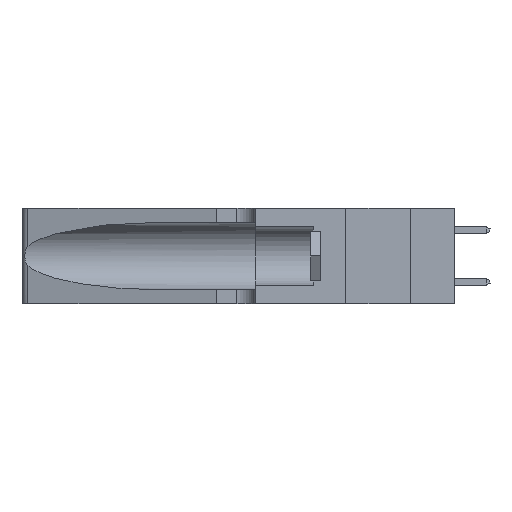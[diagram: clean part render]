
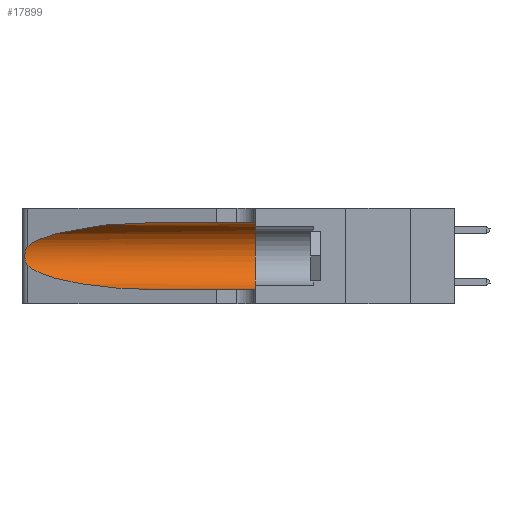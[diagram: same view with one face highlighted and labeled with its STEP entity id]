
A CAD part, left-side view. The second image highlights one B-rep face of the part: STEP entity #17899.
In plain terms, the highlighted cylindrical face has radius 3.308 mm (diameter 6.617 mm), a partial arc.
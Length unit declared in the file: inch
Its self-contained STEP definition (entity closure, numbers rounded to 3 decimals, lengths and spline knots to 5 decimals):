
#189 = DIRECTION ( 'NONE',  ( 0., 1., 0. ) ) ;
#1066 = EDGE_LOOP ( 'NONE', ( #28250, #38631, #5473, #39148, #37736, #1470 ) ) ;
#1235 = DIRECTION ( 'NONE',  ( 0., -1., 0. ) ) ;
#1470 = ORIENTED_EDGE ( 'NONE', *, *, #38438, .F. ) ;
#1581 = CARTESIAN_POINT ( 'NONE',  ( 0.2373, 1.15595, 0.08982 ) ) ;
#2326 = CARTESIAN_POINT ( 'NONE',  ( 0.25856, 1.23593, 0.16098 ) ) ;
#2476 = VERTEX_POINT ( 'NONE', #24984 ) ;
#3529 = VERTEX_POINT ( 'NONE', #33494 ) ;
#4503 = DIRECTION ( 'NONE',  ( 0., 0., -1. ) ) ;
#4847 = CARTESIAN_POINT ( 'NONE',  ( 0.1305, 0.72297, 0.05475 ) ) ;
#4878 = CARTESIAN_POINT ( 'NONE',  ( 0.1305, 0.72297, 0.31525 ) ) ;
#5461 = CARTESIAN_POINT ( 'NONE',  ( 0.25555, 1.22994, 0.2215 ) ) ;
#5473 = ORIENTED_EDGE ( 'NONE', *, *, #26069, .T. ) ;
#5600 = CARTESIAN_POINT ( 'NONE',  ( 0.25639, 1.23186, 0.15144 ) ) ;
#6011 = CARTESIAN_POINT ( 'NONE',  ( 0.1305, 1.61858, 0.05475 ) ) ;
#7937 = VERTEX_POINT ( 'NONE', #34671 ) ;
#8875 = CARTESIAN_POINT ( 'NONE',  ( 0.25487, 1.22718, 0.14631 ) ) ;
#10418 = CARTESIAN_POINT ( 'NONE',  ( 0.25487, 1.22718, 0.22369 ) ) ;
#11891 = CARTESIAN_POINT ( 'NONE',  ( 0.25639, 1.23184, 0.21858 ) ) ;
#12172 = LINE ( 'NONE', #15314, #27984 ) ;
#12780 = EDGE_CURVE ( 'NONE', #23328, #3529, #40523, .T. ) ;
#12947 = CIRCLE ( 'NONE', #27824, 0.13025 ) ;
#15090 = CARTESIAN_POINT ( 'NONE',  ( 0.25854, 1.2359, 0.20912 ) ) ;
#15314 = CARTESIAN_POINT ( 'NONE',  ( 0.1305, 1.61858, 0.31525 ) ) ;
#15371 = AXIS2_PLACEMENT_3D ( 'NONE', #26580, #1235, #4503 ) ;
#15713 = CYLINDRICAL_SURFACE ( 'NONE', #15371, 0.13025 ) ;
#17899 = ADVANCED_FACE ( 'NONE', ( #24104 ), #15713, .F. ) ;
#18194 = CARTESIAN_POINT ( 'NONE',  ( 0.1305, 0.35, 0.31525 ) ) ;
#18290 = CARTESIAN_POINT ( 'NONE',  ( 0.26075, 1.23896, 0.19203 ) ) ;
#19403 = CARTESIAN_POINT ( 'NONE',  ( 0.1305, 0.35, 0.185 ) ) ;
#19954 = CARTESIAN_POINT ( 'NONE',  ( 0.1305, 0.72297, 0.05475 ) ) ;
#20745 = VERTEX_POINT ( 'NONE', #4878 ) ;
#21445 = CARTESIAN_POINT ( 'NONE',  ( 0.26017, 1.23833, 0.17102 ) ) ;
#22554 = DIRECTION ( 'NONE',  ( 0., 0., 1. ) ) ;
#23328 = VERTEX_POINT ( 'NONE', #19954 ) ;
#23893 = CARTESIAN_POINT ( 'NONE',  ( 0.18966, 0.96281, 0.05475 ) ) ;
#24104 = FACE_OUTER_BOUND ( 'NONE', #1066, .T. ) ;
#24167 =( BOUNDED_CURVE ( )  B_SPLINE_CURVE ( 3, ( #39601, #1581, #23893, #4847 ),
 .UNSPECIFIED., .F., .F. ) 
 B_SPLINE_CURVE_WITH_KNOTS ( ( 4, 4 ),
 ( 3.44316, 4.71239 ),
 .UNSPECIFIED. ) 
 CURVE ( )  GEOMETRIC_REPRESENTATION_ITEM ( )  RATIONAL_B_SPLINE_CURVE ( ( 1., 0.87, 0.87, 1. ) ) 
 REPRESENTATION_ITEM ( '' )  );
#24605 = CARTESIAN_POINT ( 'NONE',  ( 0.25789, 1.23486, 0.15765 ) ) ;
#24984 = CARTESIAN_POINT ( 'NONE',  ( 0.25487, 1.22718, 0.14631 ) ) ;
#25215 = EDGE_CURVE ( 'NONE', #20745, #7937, #38831, .T. ) ;
#25493 = EDGE_CURVE ( 'NONE', #7937, #2476, #31513, .T. ) ;
#26069 = EDGE_CURVE ( 'NONE', #2476, #23328, #24167, .T. ) ;
#26133 = CARTESIAN_POINT ( 'NONE',  ( 0.1305, 0.72297, 0.31525 ) ) ;
#26580 = CARTESIAN_POINT ( 'NONE',  ( 0.1305, 1.61858, 0.185 ) ) ;
#27630 = CARTESIAN_POINT ( 'NONE',  ( 0.25487, 1.22718, 0.22369 ) ) ;
#27768 = CARTESIAN_POINT ( 'NONE',  ( 0.25555, 1.22993, 0.14849 ) ) ;
#27824 = AXIS2_PLACEMENT_3D ( 'NONE', #19403, #189, #22554 ) ;
#27984 = VECTOR ( 'NONE', #40545, 39.37008 ) ;
#28250 = ORIENTED_EDGE ( 'NONE', *, *, #25215, .T. ) ;
#28278 = DIRECTION ( 'NONE',  ( 0., -1., 0. ) ) ;
#29300 = CARTESIAN_POINT ( 'NONE',  ( 0.2373, 1.15595, 0.28018 ) ) ;
#30833 = EDGE_CURVE ( 'NONE', #32542, #3529, #12947, .T. ) ;
#31513 = B_SPLINE_CURVE_WITH_KNOTS ( 'NONE', 3,
 ( #27630, #5461, #11891, #34014, #15090, #37177, #18290, #40322, #21445, #2326, #24605, #5600, #27768, #8875 ),
 .UNSPECIFIED., .F., .F.,
 ( 4, 2, 2, 2, 2, 2, 4 ),
 ( 0., 0.00027, 0.00053, 0.00107, 0.0016, 0.00187, 0.00214 ),
 .UNSPECIFIED. ) ;
#32167 = VECTOR ( 'NONE', #28278, 39.37008 ) ;
#32542 = VERTEX_POINT ( 'NONE', #18194 ) ;
#33494 = CARTESIAN_POINT ( 'NONE',  ( 0.1305, 0.35, 0.05475 ) ) ;
#34014 = CARTESIAN_POINT ( 'NONE',  ( 0.25787, 1.23484, 0.2124 ) ) ;
#34671 = CARTESIAN_POINT ( 'NONE',  ( 0.25487, 1.22718, 0.22369 ) ) ;
#37177 = CARTESIAN_POINT ( 'NONE',  ( 0.26018, 1.23835, 0.19895 ) ) ;
#37736 = ORIENTED_EDGE ( 'NONE', *, *, #30833, .F. ) ;
#38438 = EDGE_CURVE ( 'NONE', #20745, #32542, #12172, .T. ) ;
#38631 = ORIENTED_EDGE ( 'NONE', *, *, #25493, .T. ) ;
#38704 = CARTESIAN_POINT ( 'NONE',  ( 0.18966, 0.96281, 0.31525 ) ) ;
#38831 =( BOUNDED_CURVE ( )  B_SPLINE_CURVE ( 3, ( #26133, #38704, #29300, #10418 ),
 .UNSPECIFIED., .F., .F. ) 
 B_SPLINE_CURVE_WITH_KNOTS ( ( 4, 4 ),
 ( 1.5708, 2.84003 ),
 .UNSPECIFIED. ) 
 CURVE ( )  GEOMETRIC_REPRESENTATION_ITEM ( )  RATIONAL_B_SPLINE_CURVE ( ( 1., 0.87, 0.87, 1. ) ) 
 REPRESENTATION_ITEM ( '' )  );
#39148 = ORIENTED_EDGE ( 'NONE', *, *, #12780, .T. ) ;
#39601 = CARTESIAN_POINT ( 'NONE',  ( 0.25487, 1.22718, 0.14631 ) ) ;
#40322 = CARTESIAN_POINT ( 'NONE',  ( 0.26075, 1.23896, 0.178 ) ) ;
#40523 = LINE ( 'NONE', #6011, #32167 ) ;
#40545 = DIRECTION ( 'NONE',  ( 0., -1., 0. ) ) ;
